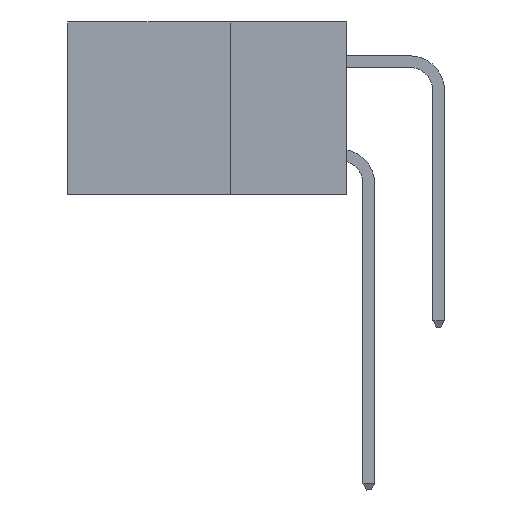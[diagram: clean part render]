
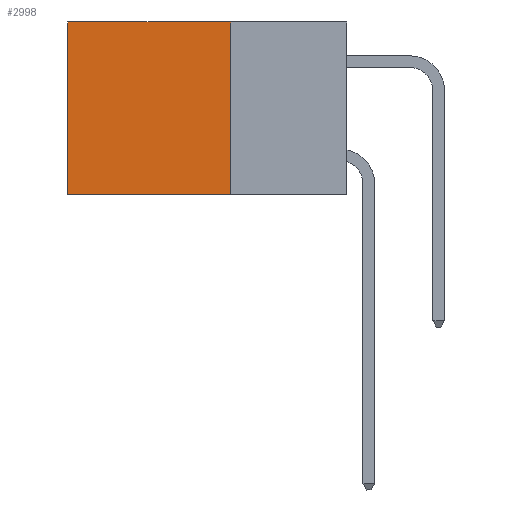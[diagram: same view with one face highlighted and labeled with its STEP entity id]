
A CAD part, left-side view. The second image highlights one B-rep face of the part: STEP entity #2998.
In plain terms, the highlighted planar face has unit normal (-1, 0, 0).
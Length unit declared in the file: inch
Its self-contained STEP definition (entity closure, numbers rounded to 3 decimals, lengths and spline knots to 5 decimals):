
#1416 = VERTEX_POINT ( 'NONE', #10559 ) ;
#1866 = VERTEX_POINT ( 'NONE', #13135 ) ;
#2109 = CARTESIAN_POINT ( 'NONE',  ( 0.2875, 0.6, 0. ) ) ;
#2593 = VERTEX_POINT ( 'NONE', #14924 ) ;
#2766 = VECTOR ( 'NONE', #9128, 39.37008 ) ;
#2998 = ADVANCED_FACE ( 'NONE', ( #12977 ), #19102, .F. ) ;
#3329 = LINE ( 'NONE', #10643, #2766 ) ;
#4385 = CARTESIAN_POINT ( 'NONE',  ( 0.2875, 0.25, -0.37 ) ) ;
#5253 = AXIS2_PLACEMENT_3D ( 'NONE', #14189, #20804, #10861 ) ;
#7390 = EDGE_LOOP ( 'NONE', ( #18872, #9428, #13204, #19597 ) ) ;
#7801 = LINE ( 'NONE', #7942, #16096 ) ;
#7942 = CARTESIAN_POINT ( 'NONE',  ( 0.2875, 0.25, -0.37 ) ) ;
#8707 = VECTOR ( 'NONE', #15485, 39.37008 ) ;
#9128 = DIRECTION ( 'NONE',  ( 0., 0., -1. ) ) ;
#9428 = ORIENTED_EDGE ( 'NONE', *, *, #19014, .F. ) ;
#10040 = CARTESIAN_POINT ( 'NONE',  ( 0.2875, 0.25, 0. ) ) ;
#10559 = CARTESIAN_POINT ( 'NONE',  ( 0.2875, 0.25, 0. ) ) ;
#10621 = EDGE_CURVE ( 'NONE', #1416, #18284, #3329, .T. ) ;
#10643 = CARTESIAN_POINT ( 'NONE',  ( 0.2875, 0.25, 0. ) ) ;
#10861 = DIRECTION ( 'NONE',  ( 0., 0., -1. ) ) ;
#11124 = LINE ( 'NONE', #10040, #19927 ) ;
#12977 = FACE_OUTER_BOUND ( 'NONE', #7390, .T. ) ;
#13135 = CARTESIAN_POINT ( 'NONE',  ( 0.2875, 0.6, -0.37 ) ) ;
#13204 = ORIENTED_EDGE ( 'NONE', *, *, #10621, .F. ) ;
#13670 = LINE ( 'NONE', #2109, #8707 ) ;
#14189 = CARTESIAN_POINT ( 'NONE',  ( 0.2875, 0.25, 0. ) ) ;
#14570 = DIRECTION ( 'NONE',  ( 0., 1., 0. ) ) ;
#14924 = CARTESIAN_POINT ( 'NONE',  ( 0.2875, 0.6, 0. ) ) ;
#15485 = DIRECTION ( 'NONE',  ( 0., 0., -1. ) ) ;
#16096 = VECTOR ( 'NONE', #14570, 39.37008 ) ;
#16840 = EDGE_CURVE ( 'NONE', #2593, #1866, #13670, .T. ) ;
#18284 = VERTEX_POINT ( 'NONE', #4385 ) ;
#18872 = ORIENTED_EDGE ( 'NONE', *, *, #16840, .T. ) ;
#19014 = EDGE_CURVE ( 'NONE', #18284, #1866, #7801, .T. ) ;
#19102 = PLANE ( 'NONE',  #5253 ) ;
#19597 = ORIENTED_EDGE ( 'NONE', *, *, #20202, .T. ) ;
#19927 = VECTOR ( 'NONE', #21630, 39.37008 ) ;
#20202 = EDGE_CURVE ( 'NONE', #1416, #2593, #11124, .T. ) ;
#20804 = DIRECTION ( 'NONE',  ( 1., 0., 0. ) ) ;
#21630 = DIRECTION ( 'NONE',  ( 0., 1., 0. ) ) ;
